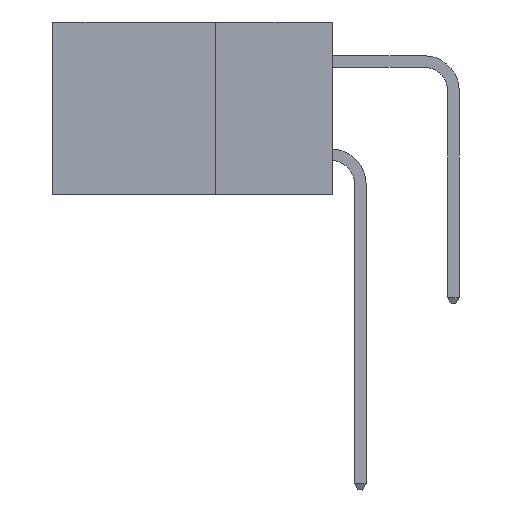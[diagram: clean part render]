
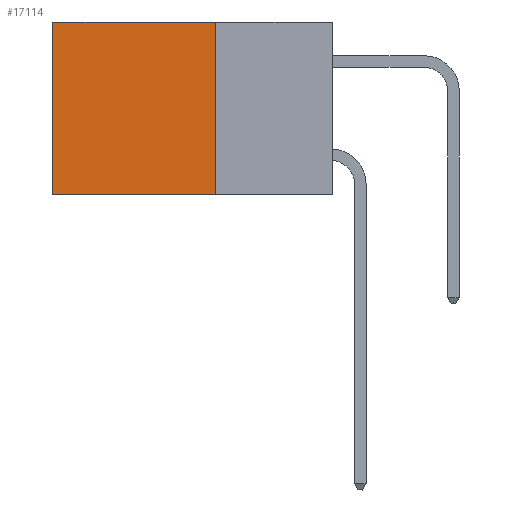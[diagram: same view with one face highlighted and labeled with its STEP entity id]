
A CAD part, left-side view. The second image highlights one B-rep face of the part: STEP entity #17114.
In plain terms, the highlighted planar face has unit normal (-1, 0, 0).
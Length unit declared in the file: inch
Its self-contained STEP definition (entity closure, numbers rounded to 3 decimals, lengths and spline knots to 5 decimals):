
#637 = CARTESIAN_POINT ( 'NONE',  ( 0.298, 0.6, -0.37 ) ) ;
#1002 = CARTESIAN_POINT ( 'NONE',  ( 0.298, 0.25, 0. ) ) ;
#1212 = LINE ( 'NONE', #1002, #9350 ) ;
#1746 = ORIENTED_EDGE ( 'NONE', *, *, #11397, .F. ) ;
#1873 = VECTOR ( 'NONE', #12619, 39.37008 ) ;
#1925 = FACE_OUTER_BOUND ( 'NONE', #7086, .T. ) ;
#2624 = DIRECTION ( 'NONE',  ( 0., 0., -1. ) ) ;
#3612 = DIRECTION ( 'NONE',  ( 1., 0., 0. ) ) ;
#4203 = EDGE_CURVE ( 'NONE', #8162, #12132, #18905, .T. ) ;
#6327 = ORIENTED_EDGE ( 'NONE', *, *, #11968, .T. ) ;
#6547 = VECTOR ( 'NONE', #10808, 39.37008 ) ;
#7086 = EDGE_LOOP ( 'NONE', ( #6327, #8249, #1746, #14727 ) ) ;
#7503 = CARTESIAN_POINT ( 'NONE',  ( 0.298, 0.25, 0. ) ) ;
#8162 = VERTEX_POINT ( 'NONE', #7503 ) ;
#8249 = ORIENTED_EDGE ( 'NONE', *, *, #11256, .F. ) ;
#9350 = VECTOR ( 'NONE', #2624, 39.37008 ) ;
#9498 = CARTESIAN_POINT ( 'NONE',  ( 0.298, 0.6, 0. ) ) ;
#10325 = CARTESIAN_POINT ( 'NONE',  ( 0.298, 0.25, -0.37 ) ) ;
#10359 = VERTEX_POINT ( 'NONE', #17794 ) ;
#10808 = DIRECTION ( 'NONE',  ( 0., 0., -1. ) ) ;
#10904 = LINE ( 'NONE', #15504, #6547 ) ;
#11256 = EDGE_CURVE ( 'NONE', #10359, #15714, #17957, .T. ) ;
#11397 = EDGE_CURVE ( 'NONE', #8162, #10359, #1212, .T. ) ;
#11758 = PLANE ( 'NONE',  #20230 ) ;
#11968 = EDGE_CURVE ( 'NONE', #12132, #15714, #10904, .T. ) ;
#12028 = DIRECTION ( 'NONE',  ( 0., 1., 0. ) ) ;
#12132 = VERTEX_POINT ( 'NONE', #9498 ) ;
#12619 = DIRECTION ( 'NONE',  ( 0., 1., 0. ) ) ;
#13324 = CARTESIAN_POINT ( 'NONE',  ( 0.298, 0.25, 0. ) ) ;
#14727 = ORIENTED_EDGE ( 'NONE', *, *, #4203, .T. ) ;
#14893 = DIRECTION ( 'NONE',  ( 0., 0., -1. ) ) ;
#15504 = CARTESIAN_POINT ( 'NONE',  ( 0.298, 0.6, 0. ) ) ;
#15714 = VERTEX_POINT ( 'NONE', #637 ) ;
#16088 = VECTOR ( 'NONE', #12028, 39.37008 ) ;
#17114 = ADVANCED_FACE ( 'NONE', ( #1925 ), #11758, .F. ) ;
#17794 = CARTESIAN_POINT ( 'NONE',  ( 0.298, 0.25, -0.37 ) ) ;
#17957 = LINE ( 'NONE', #10325, #16088 ) ;
#18905 = LINE ( 'NONE', #19624, #1873 ) ;
#19624 = CARTESIAN_POINT ( 'NONE',  ( 0.298, 0.25, 0. ) ) ;
#20230 = AXIS2_PLACEMENT_3D ( 'NONE', #13324, #3612, #14893 ) ;
